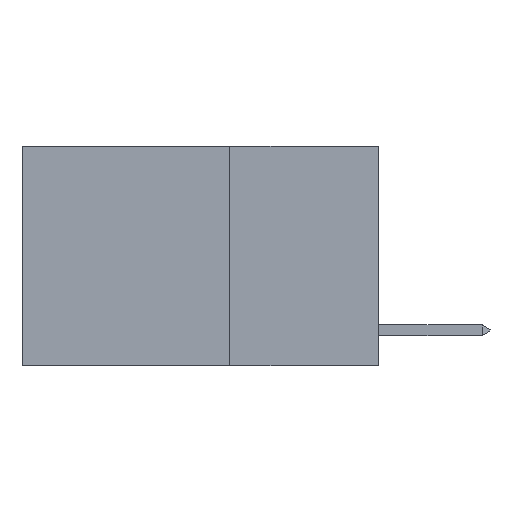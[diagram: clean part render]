
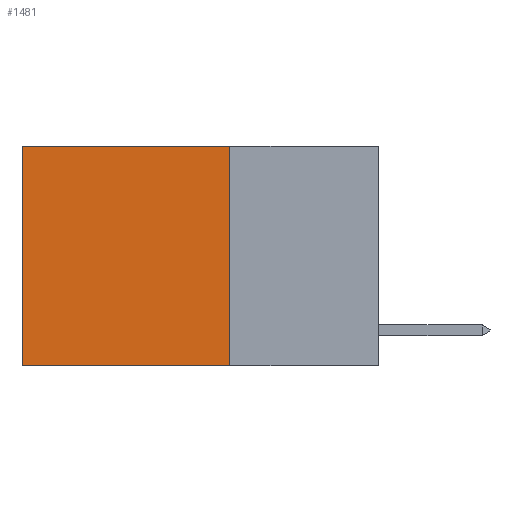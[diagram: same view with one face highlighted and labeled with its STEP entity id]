
A CAD part, left-side view. The second image highlights one B-rep face of the part: STEP entity #1481.
In plain terms, the highlighted planar face has unit normal (-1, 0, 0).
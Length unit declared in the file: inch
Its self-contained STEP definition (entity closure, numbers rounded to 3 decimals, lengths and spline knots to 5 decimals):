
#256 = ORIENTED_EDGE ( 'NONE', *, *, #8554, .T. ) ;
#428 = VERTEX_POINT ( 'NONE', #453 ) ;
#453 = CARTESIAN_POINT ( 'NONE',  ( 0.2625, 0.25, -0.37 ) ) ;
#1231 = EDGE_CURVE ( 'NONE', #6092, #4843, #1283, .T. ) ;
#1252 = AXIS2_PLACEMENT_3D ( 'NONE', #7784, #9826, #10494 ) ;
#1283 = LINE ( 'NONE', #10355, #12438 ) ;
#1481 = ADVANCED_FACE ( 'NONE', ( #6688 ), #4614, .F. ) ;
#1521 = CARTESIAN_POINT ( 'NONE',  ( 0.2625, 0.25, 0. ) ) ;
#1772 = VERTEX_POINT ( 'NONE', #2527 ) ;
#1901 = EDGE_CURVE ( 'NONE', #428, #1772, #4629, .T. ) ;
#2002 = DIRECTION ( 'NONE',  ( 0., 0., -1. ) ) ;
#2527 = CARTESIAN_POINT ( 'NONE',  ( 0.2625, 0.6, -0.37 ) ) ;
#2672 = DIRECTION ( 'NONE',  ( 0., 0., -1. ) ) ;
#2812 = VECTOR ( 'NONE', #2002, 39.37008 ) ;
#4607 = CARTESIAN_POINT ( 'NONE',  ( 0.2625, 0.25, -0.37 ) ) ;
#4614 = PLANE ( 'NONE',  #1252 ) ;
#4629 = LINE ( 'NONE', #4607, #6838 ) ;
#4843 = VERTEX_POINT ( 'NONE', #11967 ) ;
#5742 = DIRECTION ( 'NONE',  ( 0., 1., 0. ) ) ;
#5758 = LINE ( 'NONE', #11676, #2812 ) ;
#6092 = VERTEX_POINT ( 'NONE', #11948 ) ;
#6374 = ORIENTED_EDGE ( 'NONE', *, *, #1901, .F. ) ;
#6688 = FACE_OUTER_BOUND ( 'NONE', #11416, .T. ) ;
#6838 = VECTOR ( 'NONE', #5742, 39.37008 ) ;
#6949 = DIRECTION ( 'NONE',  ( 0., 1., 0. ) ) ;
#7524 = LINE ( 'NONE', #1521, #12788 ) ;
#7784 = CARTESIAN_POINT ( 'NONE',  ( 0.2625, 0.25, 0. ) ) ;
#8554 = EDGE_CURVE ( 'NONE', #4843, #1772, #5758, .T. ) ;
#9826 = DIRECTION ( 'NONE',  ( 1., 0., 0. ) ) ;
#10355 = CARTESIAN_POINT ( 'NONE',  ( 0.2625, 0.25, 0. ) ) ;
#10494 = DIRECTION ( 'NONE',  ( 0., 0., -1. ) ) ;
#11400 = EDGE_CURVE ( 'NONE', #6092, #428, #7524, .T. ) ;
#11416 = EDGE_LOOP ( 'NONE', ( #256, #6374, #13601, #12087 ) ) ;
#11676 = CARTESIAN_POINT ( 'NONE',  ( 0.2625, 0.6, 0. ) ) ;
#11948 = CARTESIAN_POINT ( 'NONE',  ( 0.2625, 0.25, 0. ) ) ;
#11967 = CARTESIAN_POINT ( 'NONE',  ( 0.2625, 0.6, 0. ) ) ;
#12087 = ORIENTED_EDGE ( 'NONE', *, *, #1231, .T. ) ;
#12438 = VECTOR ( 'NONE', #6949, 39.37008 ) ;
#12788 = VECTOR ( 'NONE', #2672, 39.37008 ) ;
#13601 = ORIENTED_EDGE ( 'NONE', *, *, #11400, .F. ) ;
